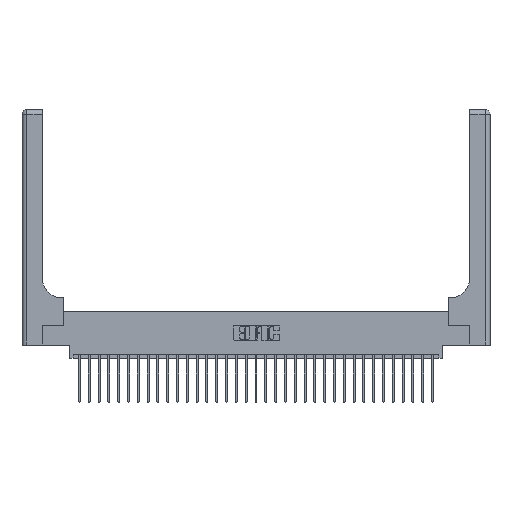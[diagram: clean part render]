
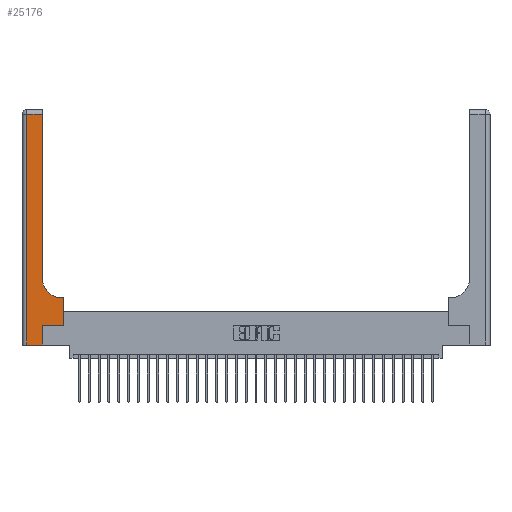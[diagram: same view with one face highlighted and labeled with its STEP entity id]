
A CAD part, top view. The second image highlights one B-rep face of the part: STEP entity #25176.
In plain terms, the highlighted planar face has unit normal (0, 0, 1).
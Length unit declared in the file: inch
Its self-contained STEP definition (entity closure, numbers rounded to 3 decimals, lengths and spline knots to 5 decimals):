
#178 = CARTESIAN_POINT ( 'NONE',  ( 0.51, 0.85, 0.37 ) ) ;
#929 = EDGE_CURVE ( 'NONE', #11280, #22534, #10777, .T. ) ;
#2770 = ORIENTED_EDGE ( 'NONE', *, *, #4905, .T. ) ;
#2774 = VECTOR ( 'NONE', #16309, 39.37008 ) ;
#3241 = EDGE_CURVE ( 'NONE', #11560, #11280, #6883, .T. ) ;
#4085 = LINE ( 'NONE', #23371, #20645 ) ;
#4229 = LINE ( 'NONE', #23047, #13331 ) ;
#4790 = LINE ( 'NONE', #12044, #28007 ) ;
#4905 = EDGE_CURVE ( 'NONE', #21229, #24063, #26753, .T. ) ;
#4971 = ORIENTED_EDGE ( 'NONE', *, *, #929, .T. ) ;
#5610 = AXIS2_PLACEMENT_3D ( 'NONE', #29542, #15297, #8357 ) ;
#5800 = EDGE_CURVE ( 'NONE', #15763, #24925, #4229, .T. ) ;
#6227 = ORIENTED_EDGE ( 'NONE', *, *, #20027, .T. ) ;
#6618 = DIRECTION ( 'NONE',  ( 0., 1., 0. ) ) ;
#6883 = LINE ( 'NONE', #13830, #2774 ) ;
#7331 = PLANE ( 'NONE',  #5610 ) ;
#7718 = VERTEX_POINT ( 'NONE', #18064 ) ;
#8054 = CARTESIAN_POINT ( 'NONE',  ( 0.265, 0.25, 0.37 ) ) ;
#8117 = DIRECTION ( 'NONE',  ( 1., 0., 0. ) ) ;
#8357 = DIRECTION ( 'NONE',  ( -1., 0., 0. ) ) ;
#9685 = DIRECTION ( 'NONE',  ( 0., 0., -1. ) ) ;
#9692 = CARTESIAN_POINT ( 'NONE',  ( 0.265, 0.25, 0.37 ) ) ;
#10777 = LINE ( 'NONE', #20032, #22691 ) ;
#11280 = VERTEX_POINT ( 'NONE', #19993 ) ;
#11560 = VERTEX_POINT ( 'NONE', #27907 ) ;
#12044 = CARTESIAN_POINT ( 'NONE',  ( 0.528, 0.25, 0.37 ) ) ;
#12540 = ORIENTED_EDGE ( 'NONE', *, *, #28796, .T. ) ;
#12563 = VERTEX_POINT ( 'NONE', #19408 ) ;
#12929 = DIRECTION ( 'NONE',  ( 1., 0., 0. ) ) ;
#12948 = AXIS2_PLACEMENT_3D ( 'NONE', #178, #9685, #8117 ) ;
#13223 = VECTOR ( 'NONE', #15149, 39.37008 ) ;
#13331 = VECTOR ( 'NONE', #13651, 39.37008 ) ;
#13651 = DIRECTION ( 'NONE',  ( -1., 0., 0. ) ) ;
#13830 = CARTESIAN_POINT ( 'NONE',  ( 0.06, 3., 0.37 ) ) ;
#14027 = EDGE_CURVE ( 'NONE', #12563, #11560, #4085, .T. ) ;
#14194 = DIRECTION ( 'NONE',  ( 0., 1., 0. ) ) ;
#15149 = DIRECTION ( 'NONE',  ( 1., 0., 0. ) ) ;
#15228 = CARTESIAN_POINT ( 'NONE',  ( 0.51, 0.6, 0.37 ) ) ;
#15297 = DIRECTION ( 'NONE',  ( 0., 0., -1. ) ) ;
#15601 = CARTESIAN_POINT ( 'NONE',  ( 0.528, 0.25, 0.37 ) ) ;
#15763 = VERTEX_POINT ( 'NONE', #16294 ) ;
#15901 = CARTESIAN_POINT ( 'NONE',  ( 0.265, 0., 0.37 ) ) ;
#16294 = CARTESIAN_POINT ( 'NONE',  ( 0.528, 0.6, 0.37 ) ) ;
#16309 = DIRECTION ( 'NONE',  ( 0., -1., 0. ) ) ;
#17109 = ORIENTED_EDGE ( 'NONE', *, *, #5800, .T. ) ;
#17398 = EDGE_CURVE ( 'NONE', #7718, #12563, #25653, .T. ) ;
#18064 = CARTESIAN_POINT ( 'NONE',  ( 0.26, 0.85, 0.37 ) ) ;
#18302 = DIRECTION ( 'NONE',  ( -1., 0., 0. ) ) ;
#18870 = ORIENTED_EDGE ( 'NONE', *, *, #3241, .T. ) ;
#19408 = CARTESIAN_POINT ( 'NONE',  ( 0.26, 2.94, 0.37 ) ) ;
#19993 = CARTESIAN_POINT ( 'NONE',  ( 0.06, 0., 0.37 ) ) ;
#20027 = EDGE_CURVE ( 'NONE', #24925, #7718, #26273, .T. ) ;
#20032 = CARTESIAN_POINT ( 'NONE',  ( 0., 0., 0.37 ) ) ;
#20083 = FACE_OUTER_BOUND ( 'NONE', #26279, .T. ) ;
#20645 = VECTOR ( 'NONE', #18302, 39.37008 ) ;
#21229 = VERTEX_POINT ( 'NONE', #9692 ) ;
#22069 = ORIENTED_EDGE ( 'NONE', *, *, #14027, .T. ) ;
#22534 = VERTEX_POINT ( 'NONE', #28645 ) ;
#22691 = VECTOR ( 'NONE', #12929, 39.37008 ) ;
#23047 = CARTESIAN_POINT ( 'NONE',  ( 0.26, 0.6, 0.37 ) ) ;
#23309 = VECTOR ( 'NONE', #6618, 39.37008 ) ;
#23371 = CARTESIAN_POINT ( 'NONE',  ( 0., 2.94, 0.37 ) ) ;
#24032 = EDGE_CURVE ( 'NONE', #22534, #21229, #25310, .T. ) ;
#24063 = VERTEX_POINT ( 'NONE', #15601 ) ;
#24925 = VERTEX_POINT ( 'NONE', #15228 ) ;
#25176 = ADVANCED_FACE ( 'NONE', ( #20083 ), #7331, .F. ) ;
#25309 = VECTOR ( 'NONE', #30044, 39.37008 ) ;
#25310 = LINE ( 'NONE', #15901, #23309 ) ;
#25548 = ORIENTED_EDGE ( 'NONE', *, *, #17398, .T. ) ;
#25653 = LINE ( 'NONE', #29897, #25309 ) ;
#25861 = ORIENTED_EDGE ( 'NONE', *, *, #24032, .T. ) ;
#26273 = CIRCLE ( 'NONE', #12948, 0.25 ) ;
#26279 = EDGE_LOOP ( 'NONE', ( #25548, #22069, #18870, #4971, #25861, #2770, #12540, #17109, #6227 ) ) ;
#26753 = LINE ( 'NONE', #8054, #13223 ) ;
#27907 = CARTESIAN_POINT ( 'NONE',  ( 0.06, 2.94, 0.37 ) ) ;
#28007 = VECTOR ( 'NONE', #14194, 39.37008 ) ;
#28645 = CARTESIAN_POINT ( 'NONE',  ( 0.265, 0., 0.37 ) ) ;
#28796 = EDGE_CURVE ( 'NONE', #24063, #15763, #4790, .T. ) ;
#29542 = CARTESIAN_POINT ( 'NONE',  ( 0., 3., 0.37 ) ) ;
#29897 = CARTESIAN_POINT ( 'NONE',  ( 0.26, 3., 0.37 ) ) ;
#30044 = DIRECTION ( 'NONE',  ( 0., 1., 0. ) ) ;
